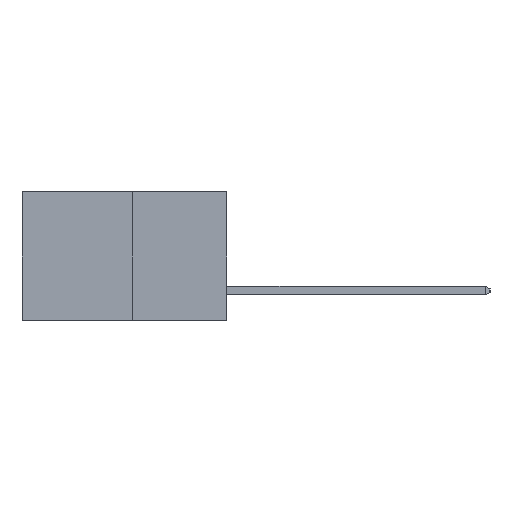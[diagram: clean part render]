
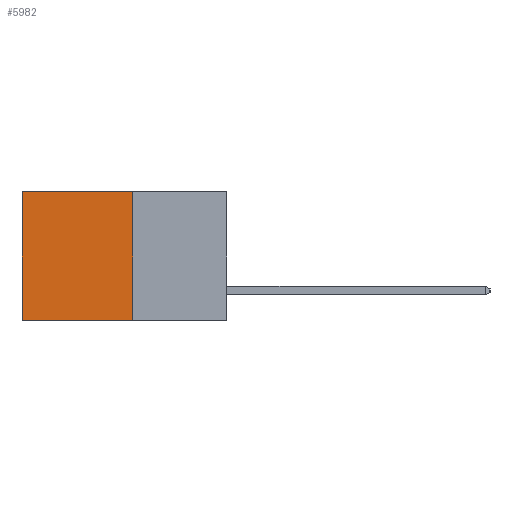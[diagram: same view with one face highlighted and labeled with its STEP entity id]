
A CAD part, left-side view. The second image highlights one B-rep face of the part: STEP entity #5982.
In plain terms, the highlighted planar face has unit normal (-1, 0, 0).
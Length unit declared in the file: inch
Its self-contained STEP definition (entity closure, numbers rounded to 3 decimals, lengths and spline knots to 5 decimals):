
#5 = DIRECTION ( 'NONE',  ( 0., 1., 0. ) ) ;
#274 = DIRECTION ( 'NONE',  ( 1., 0., 0. ) ) ;
#610 = AXIS2_PLACEMENT_3D ( 'NONE', #5397, #274, #6137 ) ;
#1567 = CARTESIAN_POINT ( 'NONE',  ( 0.277, 0.59, -0.37 ) ) ;
#2227 = ORIENTED_EDGE ( 'NONE', *, *, #8277, .F. ) ;
#2548 = EDGE_LOOP ( 'NONE', ( #8064, #9836, #2227, #4533 ) ) ;
#2731 = CARTESIAN_POINT ( 'NONE',  ( 0.277, 0.27, -0.37 ) ) ;
#2872 = EDGE_CURVE ( 'NONE', #5052, #7140, #9135, .T. ) ;
#3331 = DIRECTION ( 'NONE',  ( 0., 0., -1. ) ) ;
#3354 = VECTOR ( 'NONE', #5, 39.37008 ) ;
#3390 = LINE ( 'NONE', #6760, #7145 ) ;
#3705 = EDGE_CURVE ( 'NONE', #4170, #7140, #7005, .T. ) ;
#4170 = VERTEX_POINT ( 'NONE', #5143 ) ;
#4192 = EDGE_CURVE ( 'NONE', #9282, #4170, #6990, .T. ) ;
#4337 = CARTESIAN_POINT ( 'NONE',  ( 0.277, 0.27, -0.37 ) ) ;
#4533 = ORIENTED_EDGE ( 'NONE', *, *, #4192, .T. ) ;
#4875 = DIRECTION ( 'NONE',  ( 0., 1., 0. ) ) ;
#5052 = VERTEX_POINT ( 'NONE', #4337 ) ;
#5143 = CARTESIAN_POINT ( 'NONE',  ( 0.277, 0.59, 0. ) ) ;
#5224 = CARTESIAN_POINT ( 'NONE',  ( 0.277, 0.27, 0. ) ) ;
#5397 = CARTESIAN_POINT ( 'NONE',  ( 0.277, 0.27, -0.37 ) ) ;
#5982 = ADVANCED_FACE ( 'NONE', ( #7715 ), #9514, .F. ) ;
#6131 = CARTESIAN_POINT ( 'NONE',  ( 0.277, 0.27, 0. ) ) ;
#6137 = DIRECTION ( 'NONE',  ( 0., 0., -1. ) ) ;
#6760 = CARTESIAN_POINT ( 'NONE',  ( 0.277, 0.27, -0.37 ) ) ;
#6841 = CARTESIAN_POINT ( 'NONE',  ( 0.277, 0.59, -0.37 ) ) ;
#6990 = LINE ( 'NONE', #6131, #7190 ) ;
#7005 = LINE ( 'NONE', #1567, #7209 ) ;
#7140 = VERTEX_POINT ( 'NONE', #6841 ) ;
#7145 = VECTOR ( 'NONE', #7426, 39.37008 ) ;
#7190 = VECTOR ( 'NONE', #4875, 39.37008 ) ;
#7209 = VECTOR ( 'NONE', #3331, 39.37008 ) ;
#7426 = DIRECTION ( 'NONE',  ( 0., 0., -1. ) ) ;
#7715 = FACE_OUTER_BOUND ( 'NONE', #2548, .T. ) ;
#8064 = ORIENTED_EDGE ( 'NONE', *, *, #3705, .T. ) ;
#8277 = EDGE_CURVE ( 'NONE', #9282, #5052, #3390, .T. ) ;
#9135 = LINE ( 'NONE', #2731, #3354 ) ;
#9282 = VERTEX_POINT ( 'NONE', #5224 ) ;
#9514 = PLANE ( 'NONE',  #610 ) ;
#9836 = ORIENTED_EDGE ( 'NONE', *, *, #2872, .F. ) ;
